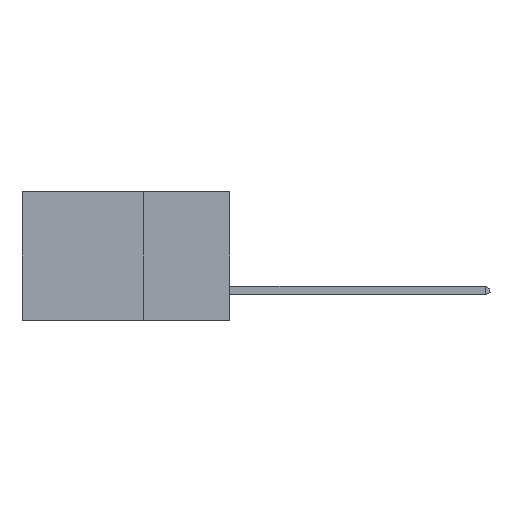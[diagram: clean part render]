
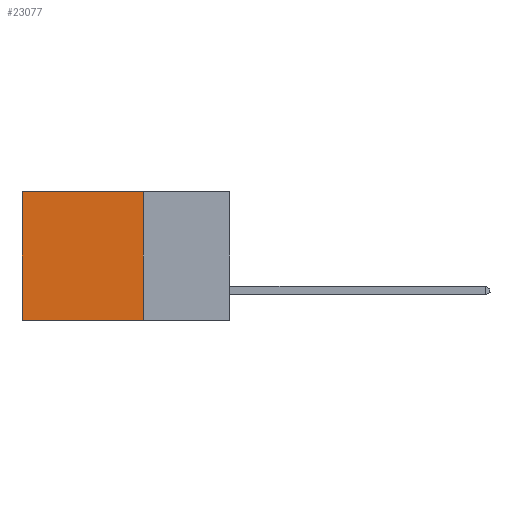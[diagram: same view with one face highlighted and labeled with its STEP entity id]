
A CAD part, left-side view. The second image highlights one B-rep face of the part: STEP entity #23077.
In plain terms, the highlighted planar face has unit normal (-1, 0, 0).
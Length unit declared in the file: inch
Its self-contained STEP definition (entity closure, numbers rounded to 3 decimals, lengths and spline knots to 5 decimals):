
#546 = LINE ( 'NONE', #11788, #11110 ) ;
#3052 = ORIENTED_EDGE ( 'NONE', *, *, #19859, .T. ) ;
#3157 = AXIS2_PLACEMENT_3D ( 'NONE', #6836, #18080, #5101 ) ;
#3181 = LINE ( 'NONE', #5575, #18784 ) ;
#3595 = CARTESIAN_POINT ( 'NONE',  ( 0.298, 0.25, 0. ) ) ;
#3813 = LINE ( 'NONE', #12785, #11150 ) ;
#3938 = VERTEX_POINT ( 'NONE', #20701 ) ;
#5101 = DIRECTION ( 'NONE',  ( 0., 0., -1. ) ) ;
#5575 = CARTESIAN_POINT ( 'NONE',  ( 0.298, 0.25, -0.37 ) ) ;
#5974 = VERTEX_POINT ( 'NONE', #21999 ) ;
#6247 = DIRECTION ( 'NONE',  ( 0., 0., -1. ) ) ;
#6836 = CARTESIAN_POINT ( 'NONE',  ( 0.298, 0.25, 0. ) ) ;
#7023 = ORIENTED_EDGE ( 'NONE', *, *, #7238, .F. ) ;
#7238 = EDGE_CURVE ( 'NONE', #11250, #19612, #546, .T. ) ;
#7256 = ORIENTED_EDGE ( 'NONE', *, *, #20831, .T. ) ;
#7492 = CARTESIAN_POINT ( 'NONE',  ( 0.298, 0.25, -0.37 ) ) ;
#7614 = VECTOR ( 'NONE', #8096, 39.37008 ) ;
#8096 = DIRECTION ( 'NONE',  ( 0., 0., -1. ) ) ;
#8667 = PLANE ( 'NONE',  #3157 ) ;
#8981 = DIRECTION ( 'NONE',  ( 0., 1., 0. ) ) ;
#11110 = VECTOR ( 'NONE', #6247, 39.37008 ) ;
#11150 = VECTOR ( 'NONE', #8981, 39.37008 ) ;
#11250 = VERTEX_POINT ( 'NONE', #3595 ) ;
#11788 = CARTESIAN_POINT ( 'NONE',  ( 0.298, 0.25, 0. ) ) ;
#12208 = EDGE_CURVE ( 'NONE', #19612, #5974, #3181, .T. ) ;
#12785 = CARTESIAN_POINT ( 'NONE',  ( 0.298, 0.25, 0. ) ) ;
#13713 = FACE_OUTER_BOUND ( 'NONE', #17985, .T. ) ;
#15354 = DIRECTION ( 'NONE',  ( 0., 1., 0. ) ) ;
#15633 = CARTESIAN_POINT ( 'NONE',  ( 0.298, 0.6, 0. ) ) ;
#17696 = LINE ( 'NONE', #15633, #7614 ) ;
#17985 = EDGE_LOOP ( 'NONE', ( #3052, #18823, #7023, #7256 ) ) ;
#18080 = DIRECTION ( 'NONE',  ( 1., 0., 0. ) ) ;
#18784 = VECTOR ( 'NONE', #15354, 39.37008 ) ;
#18823 = ORIENTED_EDGE ( 'NONE', *, *, #12208, .F. ) ;
#19612 = VERTEX_POINT ( 'NONE', #7492 ) ;
#19859 = EDGE_CURVE ( 'NONE', #3938, #5974, #17696, .T. ) ;
#20701 = CARTESIAN_POINT ( 'NONE',  ( 0.298, 0.6, 0. ) ) ;
#20831 = EDGE_CURVE ( 'NONE', #11250, #3938, #3813, .T. ) ;
#21999 = CARTESIAN_POINT ( 'NONE',  ( 0.298, 0.6, -0.37 ) ) ;
#23077 = ADVANCED_FACE ( 'NONE', ( #13713 ), #8667, .F. ) ;
